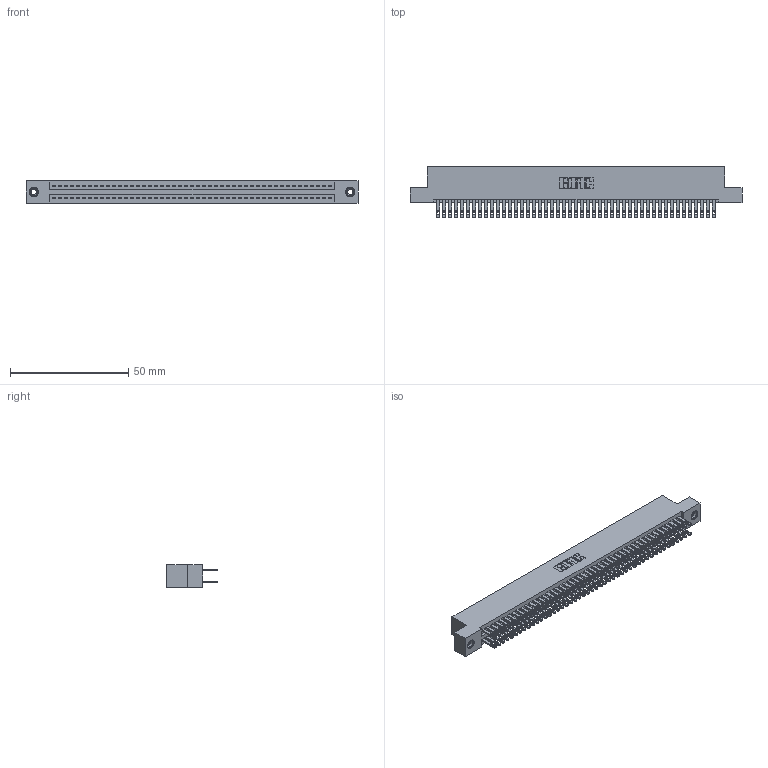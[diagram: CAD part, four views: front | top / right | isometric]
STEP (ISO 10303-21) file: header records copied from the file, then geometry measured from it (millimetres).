
FILE_DESCRIPTION (( 'STEP AP203' ), '1' );
FILE_NAME ('345-094-500-208.STEP', '2018-10-04T23:06:42', ( '' ), ( '' ), 'SwSTEP 2.0', 'SolidWorks 2016', '' );
FILE_SCHEMA (( 'CONFIG_CONTROL_DESIGN' ));
Length unit declared in the file: inch
Products named in the file (4): 345-250-001_345-250-003-102; 345-292-001_345-293-100; 345 Part_Flush Mounting Lugs - 0.156 Dia-TI; 345-094-500-208
Assembly tree (97 placements, depth 2):
  345-094-500-208
    345 Part_Flush Mounting Lugs - 0.156 Dia-TI
    345-292-001_345-293-100  x94
    345-250-001_345-250-003-102  x2
Bounding box: 140.59 x 21.51 x 9.4 mm (x, y, z)
Volume: 13984.1 mm3; surface area: 21739.9 mm2
Topology: 97 solids, 97 shells, 4510 faces, 13731 edges, 9146 vertices
Faces by surface type: plane 2650, cylinder 1844, cone 12, torus 4
Entity records: 37320 total; most frequent: CARTESIAN_POINT 6231, ORIENTED_EDGE 6158, DIRECTION 5517, EDGE_CURVE 3079, LINE 2735, VECTOR 2735, VERTEX_POINT 2048, AXIS2_PLACEMENT_3D 1391
